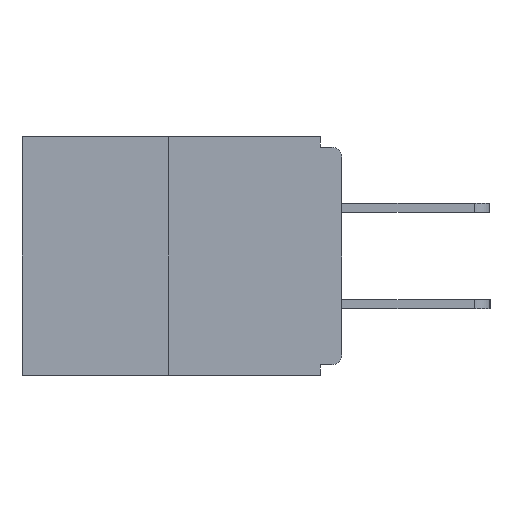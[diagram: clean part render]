
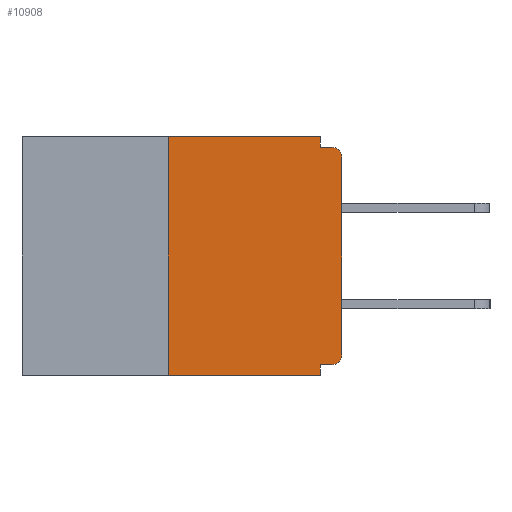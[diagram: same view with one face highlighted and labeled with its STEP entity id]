
A CAD part, left-side view. The second image highlights one B-rep face of the part: STEP entity #10908.
In plain terms, the highlighted planar face has unit normal (-1, 0, 0).
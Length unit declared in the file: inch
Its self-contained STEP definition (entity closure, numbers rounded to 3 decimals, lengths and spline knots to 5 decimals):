
#58 = VERTEX_POINT ( 'NONE', #3173 ) ;
#209 = DIRECTION ( 'NONE',  ( 0., 1., 0. ) ) ;
#271 = VERTEX_POINT ( 'NONE', #13920 ) ;
#293 = VECTOR ( 'NONE', #5594, 39.37008 ) ;
#350 = CIRCLE ( 'NONE', #14910, 0.015 ) ;
#478 = EDGE_LOOP ( 'NONE', ( #6951, #3001, #13057, #5282, #15173, #4190, #12218, #17648, #3045, #16874 ) ) ;
#1055 = AXIS2_PLACEMENT_3D ( 'NONE', #12462, #6993, #15612 ) ;
#1087 = VECTOR ( 'NONE', #209, 39.37008 ) ;
#1926 = VERTEX_POINT ( 'NONE', #17738 ) ;
#1968 = VERTEX_POINT ( 'NONE', #7030 ) ;
#2026 = EDGE_CURVE ( 'NONE', #1968, #11197, #3039, .T. ) ;
#2056 = CARTESIAN_POINT ( 'NONE',  ( 0., 0.46, -0.343 ) ) ;
#2602 = EDGE_CURVE ( 'NONE', #14665, #11157, #7578, .T. ) ;
#2610 = DIRECTION ( 'NONE',  ( -1., 0., 0. ) ) ;
#3001 = ORIENTED_EDGE ( 'NONE', *, *, #7996, .F. ) ;
#3039 = LINE ( 'NONE', #5962, #4986 ) ;
#3045 = ORIENTED_EDGE ( 'NONE', *, *, #7506, .F. ) ;
#3047 = CARTESIAN_POINT ( 'NONE',  ( 0., 0.031, 0. ) ) ;
#3173 = CARTESIAN_POINT ( 'NONE',  ( 0., 0.031, -0.015 ) ) ;
#3223 = VECTOR ( 'NONE', #4002, 39.37008 ) ;
#4002 = DIRECTION ( 'NONE',  ( 0., -1., 0. ) ) ;
#4190 = ORIENTED_EDGE ( 'NONE', *, *, #4855, .T. ) ;
#4322 = LINE ( 'NONE', #15823, #13826 ) ;
#4485 = CARTESIAN_POINT ( 'NONE',  ( 0., 0., -0.03 ) ) ;
#4735 = CARTESIAN_POINT ( 'NONE',  ( 0., 0.015, -0.015 ) ) ;
#4795 = LINE ( 'NONE', #15241, #1087 ) ;
#4855 = EDGE_CURVE ( 'NONE', #8543, #1968, #14266, .T. ) ;
#4986 = VECTOR ( 'NONE', #8810, 39.37008 ) ;
#5282 = ORIENTED_EDGE ( 'NONE', *, *, #14121, .F. ) ;
#5426 = CARTESIAN_POINT ( 'NONE',  ( 0., 0.25, 0. ) ) ;
#5436 = VERTEX_POINT ( 'NONE', #4735 ) ;
#5594 = DIRECTION ( 'NONE',  ( 0., 0., 1. ) ) ;
#5962 = CARTESIAN_POINT ( 'NONE',  ( 0., 0., 0. ) ) ;
#6168 = AXIS2_PLACEMENT_3D ( 'NONE', #15123, #6862, #16305 ) ;
#6248 = VECTOR ( 'NONE', #14555, 39.37008 ) ;
#6580 = CARTESIAN_POINT ( 'NONE',  ( 0., 0.031, -0.328 ) ) ;
#6799 = DIRECTION ( 'NONE',  ( 0., 0., -1. ) ) ;
#6862 = DIRECTION ( 'NONE',  ( -1., 0., 0. ) ) ;
#6951 = ORIENTED_EDGE ( 'NONE', *, *, #2602, .F. ) ;
#6993 = DIRECTION ( 'NONE',  ( 1., 0., 0. ) ) ;
#7030 = CARTESIAN_POINT ( 'NONE',  ( 0., 0., -0.313 ) ) ;
#7103 = LINE ( 'NONE', #3047, #14848 ) ;
#7297 = LINE ( 'NONE', #5426, #293 ) ;
#7344 = FACE_OUTER_BOUND ( 'NONE', #478, .T. ) ;
#7396 = CARTESIAN_POINT ( 'NONE',  ( 0., 0.46, 0. ) ) ;
#7506 = EDGE_CURVE ( 'NONE', #58, #5436, #11445, .T. ) ;
#7578 = LINE ( 'NONE', #7396, #9107 ) ;
#7637 = EDGE_CURVE ( 'NONE', #11157, #58, #7103, .T. ) ;
#7996 = EDGE_CURVE ( 'NONE', #271, #14665, #7297, .T. ) ;
#8269 = CARTESIAN_POINT ( 'NONE',  ( 0., 0.031, 0. ) ) ;
#8543 = VERTEX_POINT ( 'NONE', #15615 ) ;
#8810 = DIRECTION ( 'NONE',  ( 0., 0., 1. ) ) ;
#8828 = EDGE_CURVE ( 'NONE', #11197, #5436, #350, .T. ) ;
#9107 = VECTOR ( 'NONE', #12727, 39.37008 ) ;
#10165 = DIRECTION ( 'NONE',  ( 0., 0., -1. ) ) ;
#10657 = EDGE_CURVE ( 'NONE', #8543, #11064, #4795, .T. ) ;
#10908 = ADVANCED_FACE ( 'NONE', ( #7344 ), #15262, .F. ) ;
#10934 = CARTESIAN_POINT ( 'NONE',  ( 0., 0.015, -0.03 ) ) ;
#11064 = VERTEX_POINT ( 'NONE', #6580 ) ;
#11157 = VERTEX_POINT ( 'NONE', #8269 ) ;
#11197 = VERTEX_POINT ( 'NONE', #4485 ) ;
#11445 = LINE ( 'NONE', #17824, #3223 ) ;
#12218 = ORIENTED_EDGE ( 'NONE', *, *, #2026, .T. ) ;
#12462 = CARTESIAN_POINT ( 'NONE',  ( 0., 0.46, 0. ) ) ;
#12727 = DIRECTION ( 'NONE',  ( 0., -1., 0. ) ) ;
#13057 = ORIENTED_EDGE ( 'NONE', *, *, #13079, .T. ) ;
#13079 = EDGE_CURVE ( 'NONE', #271, #1926, #17312, .T. ) ;
#13826 = VECTOR ( 'NONE', #10165, 39.37008 ) ;
#13920 = CARTESIAN_POINT ( 'NONE',  ( 0., 0.25, -0.343 ) ) ;
#14121 = EDGE_CURVE ( 'NONE', #11064, #1926, #4322, .T. ) ;
#14266 = CIRCLE ( 'NONE', #6168, 0.015 ) ;
#14555 = DIRECTION ( 'NONE',  ( 0., -1., 0. ) ) ;
#14665 = VERTEX_POINT ( 'NONE', #14932 ) ;
#14848 = VECTOR ( 'NONE', #16815, 39.37008 ) ;
#14910 = AXIS2_PLACEMENT_3D ( 'NONE', #10934, #2610, #6799 ) ;
#14932 = CARTESIAN_POINT ( 'NONE',  ( 0., 0.25, 0. ) ) ;
#15123 = CARTESIAN_POINT ( 'NONE',  ( 0., 0.015, -0.313 ) ) ;
#15173 = ORIENTED_EDGE ( 'NONE', *, *, #10657, .F. ) ;
#15241 = CARTESIAN_POINT ( 'NONE',  ( 0., 0., -0.328 ) ) ;
#15262 = PLANE ( 'NONE',  #1055 ) ;
#15612 = DIRECTION ( 'NONE',  ( 0., 0., -1. ) ) ;
#15615 = CARTESIAN_POINT ( 'NONE',  ( 0., 0.015, -0.328 ) ) ;
#15823 = CARTESIAN_POINT ( 'NONE',  ( 0., 0.031, -0.343 ) ) ;
#16305 = DIRECTION ( 'NONE',  ( 0., 0., -1. ) ) ;
#16815 = DIRECTION ( 'NONE',  ( 0., 0., -1. ) ) ;
#16874 = ORIENTED_EDGE ( 'NONE', *, *, #7637, .F. ) ;
#17312 = LINE ( 'NONE', #2056, #6248 ) ;
#17648 = ORIENTED_EDGE ( 'NONE', *, *, #8828, .T. ) ;
#17738 = CARTESIAN_POINT ( 'NONE',  ( 0., 0.031, -0.343 ) ) ;
#17824 = CARTESIAN_POINT ( 'NONE',  ( 0., 0., -0.015 ) ) ;
